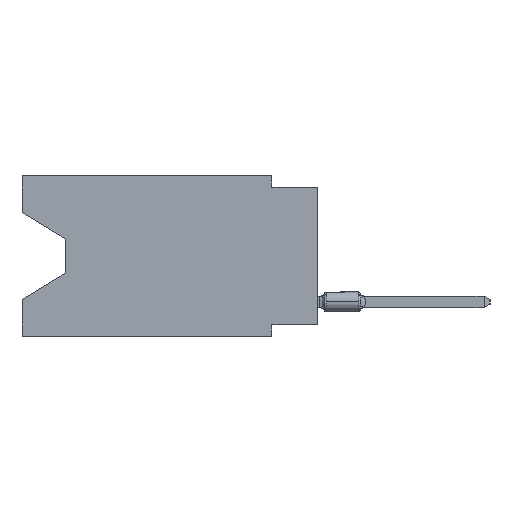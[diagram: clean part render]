
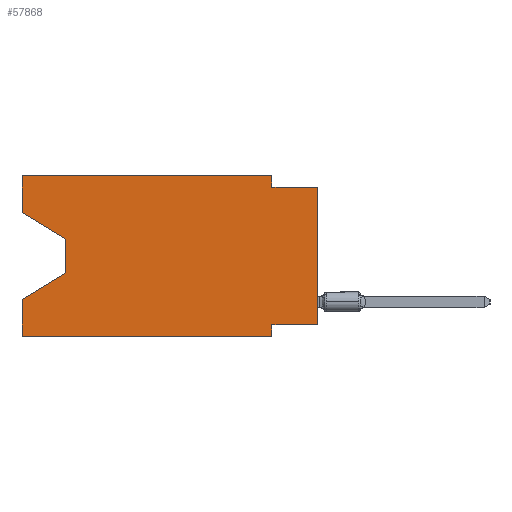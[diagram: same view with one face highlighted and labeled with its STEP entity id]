
A CAD part, left-side view. The second image highlights one B-rep face of the part: STEP entity #57868.
In plain terms, the highlighted planar face has unit normal (-1, 0, 0).
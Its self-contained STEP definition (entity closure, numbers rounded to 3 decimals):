
#582 = DIRECTION ( 'NONE',  ( 0., 0., 1. ) ) ;
#704 = CARTESIAN_POINT ( 'NONE',  ( 0., 0., -0.635 ) ) ;
#779 = LINE ( 'NONE', #5796, #4814 ) ;
#1031 = VERTEX_POINT ( 'NONE', #34216 ) ;
#1996 = ORIENTED_EDGE ( 'NONE', *, *, #19484, .F. ) ;
#3384 = DIRECTION ( 'NONE',  ( 0., -0.855, -0.519 ) ) ;
#4331 = CARTESIAN_POINT ( 'NONE',  ( 0., 13.97, -5.385 ) ) ;
#4531 = VERTEX_POINT ( 'NONE', #12821 ) ;
#4814 = VECTOR ( 'NONE', #36530, 1000. ) ;
#4990 = VERTEX_POINT ( 'NONE', #63193 ) ;
#5062 = EDGE_LOOP ( 'NONE', ( #28014, #37163, #31652, #53346, #52031, #41213, #58462, #43661, #1996, #28368, #20603, #57282 ) ) ;
#5796 = CARTESIAN_POINT ( 'NONE',  ( 0., 13.97, -3.505 ) ) ;
#5976 = DIRECTION ( 'NONE',  ( 0., -1., 0. ) ) ;
#7131 = VERTEX_POINT ( 'NONE', #24057 ) ;
#7600 = VERTEX_POINT ( 'NONE', #35427 ) ;
#8067 = VECTOR ( 'NONE', #42165, 1000. ) ;
#8364 = EDGE_CURVE ( 'NONE', #12602, #25414, #41421, .T. ) ;
#9382 = CARTESIAN_POINT ( 'NONE',  ( 0., 13.97, -3.505 ) ) ;
#12435 = CARTESIAN_POINT ( 'NONE',  ( 0., 16.383, 0. ) ) ;
#12602 = VERTEX_POINT ( 'NONE', #56962 ) ;
#12821 = CARTESIAN_POINT ( 'NONE',  ( 0., 16.383, 0. ) ) ;
#12914 = VECTOR ( 'NONE', #27540, 1000. ) ;
#14890 = VECTOR ( 'NONE', #22567, 1000. ) ;
#17192 = CARTESIAN_POINT ( 'NONE',  ( 0., 2.54, 0. ) ) ;
#17237 = CARTESIAN_POINT ( 'NONE',  ( 0., 0., -8.255 ) ) ;
#19484 = EDGE_CURVE ( 'NONE', #63794, #46972, #35797, .T. ) ;
#20419 = CARTESIAN_POINT ( 'NONE',  ( 0., 2.54, -8.89 ) ) ;
#20603 = ORIENTED_EDGE ( 'NONE', *, *, #40594, .F. ) ;
#22567 = DIRECTION ( 'NONE',  ( 0., 1., 0. ) ) ;
#22820 = EDGE_CURVE ( 'NONE', #1031, #60200, #65175, .T. ) ;
#22978 = VECTOR ( 'NONE', #40782, 1000. ) ;
#24057 = CARTESIAN_POINT ( 'NONE',  ( 0., 0., -8.255 ) ) ;
#25414 = VERTEX_POINT ( 'NONE', #25634 ) ;
#25634 = CARTESIAN_POINT ( 'NONE',  ( 0., 2.54, -8.89 ) ) ;
#26068 = EDGE_CURVE ( 'NONE', #61740, #1031, #779, .T. ) ;
#26659 = LINE ( 'NONE', #36654, #36659 ) ;
#27540 = DIRECTION ( 'NONE',  ( 0., 0., -1. ) ) ;
#27827 = LINE ( 'NONE', #12435, #8067 ) ;
#28014 = ORIENTED_EDGE ( 'NONE', *, *, #51076, .T. ) ;
#28368 = ORIENTED_EDGE ( 'NONE', *, *, #52415, .F. ) ;
#29335 = VERTEX_POINT ( 'NONE', #40706 ) ;
#30769 = LINE ( 'NONE', #50837, #51563 ) ;
#30878 = DIRECTION ( 'NONE',  ( 1., 0., 0. ) ) ;
#31652 = ORIENTED_EDGE ( 'NONE', *, *, #22820, .T. ) ;
#31997 = EDGE_CURVE ( 'NONE', #7131, #12602, #44186, .T. ) ;
#33779 = CARTESIAN_POINT ( 'NONE',  ( 0., 16.383, -2.038 ) ) ;
#34216 = CARTESIAN_POINT ( 'NONE',  ( 0., 13.97, -5.385 ) ) ;
#35427 = CARTESIAN_POINT ( 'NONE',  ( 0., 2.54, 0. ) ) ;
#35797 = LINE ( 'NONE', #704, #54424 ) ;
#35953 = CARTESIAN_POINT ( 'NONE',  ( 0., 16.383, -6.852 ) ) ;
#36530 = DIRECTION ( 'NONE',  ( 0., 0., -1. ) ) ;
#36654 = CARTESIAN_POINT ( 'NONE',  ( 0., 16.383, 0. ) ) ;
#36659 = VECTOR ( 'NONE', #62067, 1000. ) ;
#36925 = CARTESIAN_POINT ( 'NONE',  ( 0., 0., -0.635 ) ) ;
#37163 = ORIENTED_EDGE ( 'NONE', *, *, #26068, .T. ) ;
#37218 = FACE_OUTER_BOUND ( 'NONE', #5062, .T. ) ;
#37546 = LINE ( 'NONE', #17192, #12914 ) ;
#39645 = CARTESIAN_POINT ( 'NONE',  ( 0., 2.54, -0.635 ) ) ;
#40594 = EDGE_CURVE ( 'NONE', #4531, #7600, #26659, .T. ) ;
#40706 = CARTESIAN_POINT ( 'NONE',  ( 0., 16.383, -2.038 ) ) ;
#40782 = DIRECTION ( 'NONE',  ( 0., 0., -1. ) ) ;
#40960 = VECTOR ( 'NONE', #59831, 1000. ) ;
#41213 = ORIENTED_EDGE ( 'NONE', *, *, #8364, .F. ) ;
#41421 = LINE ( 'NONE', #20419, #22978 ) ;
#41548 = PLANE ( 'NONE',  #45140 ) ;
#41677 = LINE ( 'NONE', #61732, #49713 ) ;
#42165 = DIRECTION ( 'NONE',  ( 0., 0., 1. ) ) ;
#43661 = ORIENTED_EDGE ( 'NONE', *, *, #49586, .T. ) ;
#44186 = LINE ( 'NONE', #17237, #14890 ) ;
#44472 = LINE ( 'NONE', #33779, #48023 ) ;
#45140 = AXIS2_PLACEMENT_3D ( 'NONE', #51938, #30878, #57291 ) ;
#45161 = DIRECTION ( 'NONE',  ( 0., 0., 1. ) ) ;
#46680 = EDGE_CURVE ( 'NONE', #29335, #4531, #27827, .T. ) ;
#46972 = VERTEX_POINT ( 'NONE', #36925 ) ;
#48023 = VECTOR ( 'NONE', #3384, 1000. ) ;
#49586 = EDGE_CURVE ( 'NONE', #7131, #46972, #30769, .T. ) ;
#49713 = VECTOR ( 'NONE', #582, 1000. ) ;
#50837 = CARTESIAN_POINT ( 'NONE',  ( 0., 0., 0. ) ) ;
#51076 = EDGE_CURVE ( 'NONE', #29335, #61740, #44472, .T. ) ;
#51563 = VECTOR ( 'NONE', #45161, 1000. ) ;
#51770 = CARTESIAN_POINT ( 'NONE',  ( 0., 16.383, -8.89 ) ) ;
#51845 = DIRECTION ( 'NONE',  ( 0., -1., 0. ) ) ;
#51938 = CARTESIAN_POINT ( 'NONE',  ( 0., 16.383, 0. ) ) ;
#52031 = ORIENTED_EDGE ( 'NONE', *, *, #58732, .T. ) ;
#52415 = EDGE_CURVE ( 'NONE', #7600, #63794, #37546, .T. ) ;
#53346 = ORIENTED_EDGE ( 'NONE', *, *, #62413, .F. ) ;
#54424 = VECTOR ( 'NONE', #51845, 1000. ) ;
#56785 = LINE ( 'NONE', #51770, #64469 ) ;
#56962 = CARTESIAN_POINT ( 'NONE',  ( 0., 2.54, -8.255 ) ) ;
#57282 = ORIENTED_EDGE ( 'NONE', *, *, #46680, .F. ) ;
#57291 = DIRECTION ( 'NONE',  ( 0., 0., -1. ) ) ;
#57868 = ADVANCED_FACE ( 'NONE', ( #37218 ), #41548, .F. ) ;
#58462 = ORIENTED_EDGE ( 'NONE', *, *, #31997, .F. ) ;
#58732 = EDGE_CURVE ( 'NONE', #4990, #25414, #56785, .T. ) ;
#59831 = DIRECTION ( 'NONE',  ( 0., 0.855, -0.519 ) ) ;
#60200 = VERTEX_POINT ( 'NONE', #35953 ) ;
#61732 = CARTESIAN_POINT ( 'NONE',  ( 0., 16.383, 0. ) ) ;
#61740 = VERTEX_POINT ( 'NONE', #9382 ) ;
#62067 = DIRECTION ( 'NONE',  ( 0., -1., 0. ) ) ;
#62413 = EDGE_CURVE ( 'NONE', #4990, #60200, #41677, .T. ) ;
#63193 = CARTESIAN_POINT ( 'NONE',  ( 0., 16.383, -8.89 ) ) ;
#63794 = VERTEX_POINT ( 'NONE', #39645 ) ;
#64469 = VECTOR ( 'NONE', #5976, 1000. ) ;
#65175 = LINE ( 'NONE', #4331, #40960 ) ;
